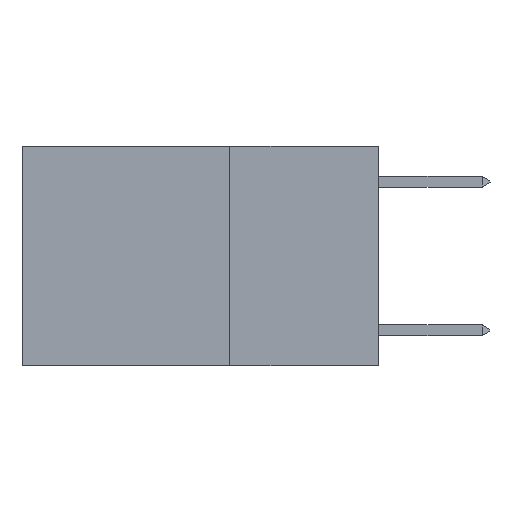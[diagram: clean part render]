
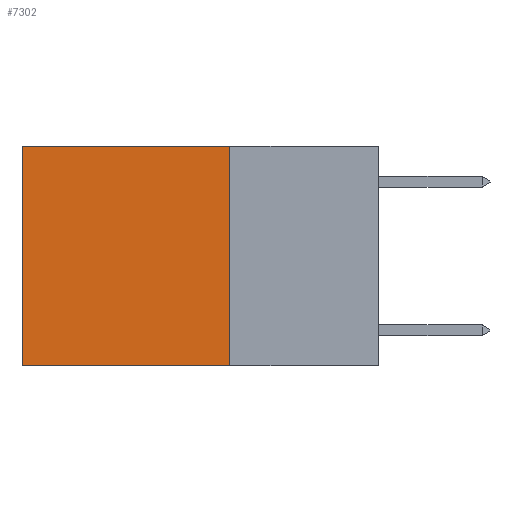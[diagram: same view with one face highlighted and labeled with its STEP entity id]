
A CAD part, left-side view. The second image highlights one B-rep face of the part: STEP entity #7302.
In plain terms, the highlighted planar face has unit normal (-1, 0, 0).
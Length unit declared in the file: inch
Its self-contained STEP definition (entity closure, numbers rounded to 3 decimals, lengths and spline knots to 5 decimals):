
#1057 = DIRECTION ( 'NONE',  ( 1., 0., 0. ) ) ;
#1873 = DIRECTION ( 'NONE',  ( 0., 1., 0. ) ) ;
#2223 = CARTESIAN_POINT ( 'NONE',  ( 0.2625, 0.25, 0. ) ) ;
#2313 = VERTEX_POINT ( 'NONE', #30734 ) ;
#4664 = ORIENTED_EDGE ( 'NONE', *, *, #10376, .T. ) ;
#7242 = CARTESIAN_POINT ( 'NONE',  ( 0.2625, 0.25, -0.37 ) ) ;
#7302 = ADVANCED_FACE ( 'NONE', ( #19674 ), #17618, .F. ) ;
#7528 = ORIENTED_EDGE ( 'NONE', *, *, #14035, .F. ) ;
#7811 = CARTESIAN_POINT ( 'NONE',  ( 0.2625, 0.25, -0.37 ) ) ;
#8163 = CARTESIAN_POINT ( 'NONE',  ( 0.2625, 0.6, -0.37 ) ) ;
#8601 = DIRECTION ( 'NONE',  ( 0., 0., -1. ) ) ;
#8700 = EDGE_CURVE ( 'NONE', #2313, #29662, #28609, .T. ) ;
#8978 = EDGE_LOOP ( 'NONE', ( #27859, #11864, #7528, #4664 ) ) ;
#10376 = EDGE_CURVE ( 'NONE', #17534, #2313, #11308, .T. ) ;
#10663 = AXIS2_PLACEMENT_3D ( 'NONE', #19835, #1057, #29408 ) ;
#11308 = LINE ( 'NONE', #20905, #18727 ) ;
#11317 = EDGE_CURVE ( 'NONE', #30535, #29662, #25959, .T. ) ;
#11864 = ORIENTED_EDGE ( 'NONE', *, *, #11317, .F. ) ;
#11951 = CARTESIAN_POINT ( 'NONE',  ( 0.2625, 0.6, 0. ) ) ;
#14035 = EDGE_CURVE ( 'NONE', #17534, #30535, #23087, .T. ) ;
#17534 = VERTEX_POINT ( 'NONE', #2223 ) ;
#17618 = PLANE ( 'NONE',  #10663 ) ;
#18727 = VECTOR ( 'NONE', #23569, 39.37008 ) ;
#19674 = FACE_OUTER_BOUND ( 'NONE', #8978, .T. ) ;
#19835 = CARTESIAN_POINT ( 'NONE',  ( 0.2625, 0.25, 0. ) ) ;
#20905 = CARTESIAN_POINT ( 'NONE',  ( 0.2625, 0.25, 0. ) ) ;
#22194 = DIRECTION ( 'NONE',  ( 0., 0., -1. ) ) ;
#22582 = VECTOR ( 'NONE', #22194, 39.37008 ) ;
#23087 = LINE ( 'NONE', #25590, #23190 ) ;
#23190 = VECTOR ( 'NONE', #8601, 39.37008 ) ;
#23569 = DIRECTION ( 'NONE',  ( 0., 1., 0. ) ) ;
#25590 = CARTESIAN_POINT ( 'NONE',  ( 0.2625, 0.25, 0. ) ) ;
#25959 = LINE ( 'NONE', #7242, #27416 ) ;
#27416 = VECTOR ( 'NONE', #1873, 39.37008 ) ;
#27859 = ORIENTED_EDGE ( 'NONE', *, *, #8700, .T. ) ;
#28609 = LINE ( 'NONE', #11951, #22582 ) ;
#29408 = DIRECTION ( 'NONE',  ( 0., 0., -1. ) ) ;
#29662 = VERTEX_POINT ( 'NONE', #8163 ) ;
#30535 = VERTEX_POINT ( 'NONE', #7811 ) ;
#30734 = CARTESIAN_POINT ( 'NONE',  ( 0.2625, 0.6, 0. ) ) ;
